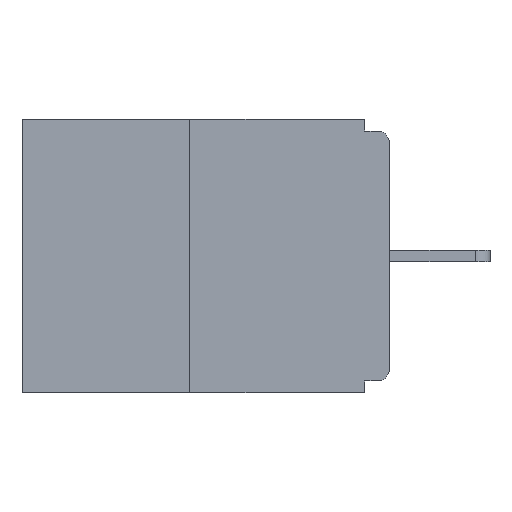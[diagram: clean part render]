
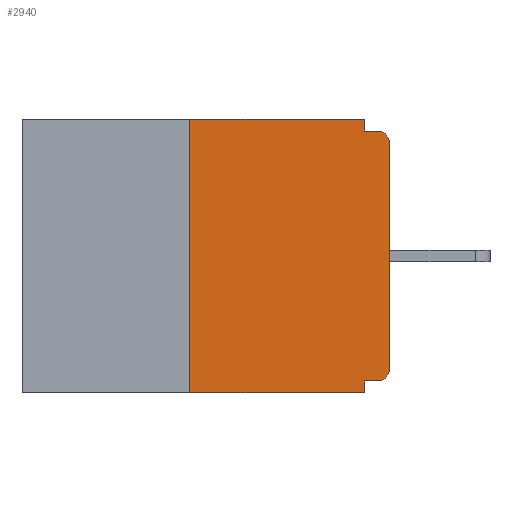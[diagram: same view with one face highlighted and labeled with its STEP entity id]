
A CAD part, left-side view. The second image highlights one B-rep face of the part: STEP entity #2940.
In plain terms, the highlighted planar face has unit normal (-1, 0, 0).
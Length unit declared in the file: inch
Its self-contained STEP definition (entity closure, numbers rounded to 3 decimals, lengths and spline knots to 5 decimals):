
#177 = FACE_OUTER_BOUND ( 'NONE', #659, .T. ) ;
#199 = CARTESIAN_POINT ( 'NONE',  ( 0., 0.015, -0.328 ) ) ;
#419 = CARTESIAN_POINT ( 'NONE',  ( 0., 0.031, 0. ) ) ;
#659 = EDGE_LOOP ( 'NONE', ( #4234, #4294, #4307, #4399, #4528, #4641, #4643, #4675, #4744, #4788 ) ) ;
#660 = VECTOR ( 'NONE', #5358, 39.37008 ) ;
#672 = VECTOR ( 'NONE', #8830, 39.37008 ) ;
#677 = LINE ( 'NONE', #7534, #672 ) ;
#694 = LINE ( 'NONE', #4751, #660 ) ;
#746 = VECTOR ( 'NONE', #3418, 39.37008 ) ;
#864 = LINE ( 'NONE', #7514, #746 ) ;
#878 = VECTOR ( 'NONE', #9875, 39.37008 ) ;
#987 = AXIS2_PLACEMENT_3D ( 'NONE', #4759, #5664, #1078 ) ;
#1072 = LINE ( 'NONE', #3291, #878 ) ;
#1078 = DIRECTION ( 'NONE',  ( 0., 0., -1. ) ) ;
#1327 = PLANE ( 'NONE',  #10338 ) ;
#1788 = VERTEX_POINT ( 'NONE', #419 ) ;
#1870 = EDGE_CURVE ( 'NONE', #2166, #1788, #6035, .T. ) ;
#2054 = EDGE_CURVE ( 'NONE', #8204, #8087, #4799, .T. ) ;
#2150 = EDGE_CURVE ( 'NONE', #7893, #8150, #4353, .T. ) ;
#2166 = VERTEX_POINT ( 'NONE', #4465 ) ;
#2228 = EDGE_CURVE ( 'NONE', #7756, #8025, #4148, .T. ) ;
#2294 = EDGE_CURVE ( 'NONE', #7893, #8204, #3614, .T. ) ;
#2298 = CARTESIAN_POINT ( 'NONE',  ( 0., 0., -0.328 ) ) ;
#2368 = EDGE_CURVE ( 'NONE', #8087, #8025, #3404, .T. ) ;
#2396 = DIRECTION ( 'NONE',  ( 0., -1., 0. ) ) ;
#2397 = CARTESIAN_POINT ( 'NONE',  ( 0., 0.46, 0. ) ) ;
#2735 = CARTESIAN_POINT ( 'NONE',  ( 0., 0.031, -0.015 ) ) ;
#2753 = EDGE_CURVE ( 'NONE', #7722, #2166, #1072, .T. ) ;
#2779 = EDGE_CURVE ( 'NONE', #7722, #3634, #864, .T. ) ;
#2795 = EDGE_CURVE ( 'NONE', #8150, #3634, #677, .T. ) ;
#2811 = EDGE_CURVE ( 'NONE', #1788, #7756, #694, .T. ) ;
#2940 = ADVANCED_FACE ( 'NONE', ( #177 ), #1327, .F. ) ;
#3130 = CARTESIAN_POINT ( 'NONE',  ( 0., 0.25, -0.343 ) ) ;
#3291 = CARTESIAN_POINT ( 'NONE',  ( 0., 0.25, 0. ) ) ;
#3404 = CIRCLE ( 'NONE', #987, 0.015 ) ;
#3418 = DIRECTION ( 'NONE',  ( 0., -1., 0. ) ) ;
#3599 = DIRECTION ( 'NONE',  ( 0., 1., 0. ) ) ;
#3601 = CARTESIAN_POINT ( 'NONE',  ( 0., 0., -0.313 ) ) ;
#3614 = CIRCLE ( 'NONE', #9066, 0.015 ) ;
#3634 = VERTEX_POINT ( 'NONE', #5076 ) ;
#3985 = VECTOR ( 'NONE', #5439, 39.37008 ) ;
#4148 = LINE ( 'NONE', #5165, #3985 ) ;
#4234 = ORIENTED_EDGE ( 'NONE', *, *, #1870, .F. ) ;
#4284 = VECTOR ( 'NONE', #3599, 39.37008 ) ;
#4294 = ORIENTED_EDGE ( 'NONE', *, *, #2753, .F. ) ;
#4307 = ORIENTED_EDGE ( 'NONE', *, *, #2779, .T. ) ;
#4353 = LINE ( 'NONE', #2298, #4284 ) ;
#4399 = ORIENTED_EDGE ( 'NONE', *, *, #2795, .F. ) ;
#4465 = CARTESIAN_POINT ( 'NONE',  ( 0., 0.25, 0. ) ) ;
#4528 = ORIENTED_EDGE ( 'NONE', *, *, #2150, .F. ) ;
#4636 = DIRECTION ( 'NONE',  ( 1., 0., 0. ) ) ;
#4641 = ORIENTED_EDGE ( 'NONE', *, *, #2294, .T. ) ;
#4643 = ORIENTED_EDGE ( 'NONE', *, *, #2054, .T. ) ;
#4675 = ORIENTED_EDGE ( 'NONE', *, *, #2368, .T. ) ;
#4744 = ORIENTED_EDGE ( 'NONE', *, *, #2228, .F. ) ;
#4751 = CARTESIAN_POINT ( 'NONE',  ( 0., 0.031, 0. ) ) ;
#4759 = CARTESIAN_POINT ( 'NONE',  ( 0., 0.015, -0.03 ) ) ;
#4788 = ORIENTED_EDGE ( 'NONE', *, *, #2811, .F. ) ;
#4799 = LINE ( 'NONE', #7427, #5336 ) ;
#5076 = CARTESIAN_POINT ( 'NONE',  ( 0., 0.031, -0.343 ) ) ;
#5165 = CARTESIAN_POINT ( 'NONE',  ( 0., 0., -0.015 ) ) ;
#5200 = CARTESIAN_POINT ( 'NONE',  ( 0., 0., -0.03 ) ) ;
#5336 = VECTOR ( 'NONE', #6385, 39.37008 ) ;
#5358 = DIRECTION ( 'NONE',  ( 0., 0., -1. ) ) ;
#5439 = DIRECTION ( 'NONE',  ( 0., -1., 0. ) ) ;
#5664 = DIRECTION ( 'NONE',  ( -1., 0., 0. ) ) ;
#6035 = LINE ( 'NONE', #2397, #6055 ) ;
#6055 = VECTOR ( 'NONE', #2396, 39.37008 ) ;
#6385 = DIRECTION ( 'NONE',  ( 0., 0., 1. ) ) ;
#6772 = DIRECTION ( 'NONE',  ( 0., 0., -1. ) ) ;
#7427 = CARTESIAN_POINT ( 'NONE',  ( 0., 0., 0. ) ) ;
#7514 = CARTESIAN_POINT ( 'NONE',  ( 0., 0.46, -0.343 ) ) ;
#7534 = CARTESIAN_POINT ( 'NONE',  ( 0., 0.031, -0.343 ) ) ;
#7722 = VERTEX_POINT ( 'NONE', #3130 ) ;
#7756 = VERTEX_POINT ( 'NONE', #2735 ) ;
#7888 = DIRECTION ( 'NONE',  ( 0., 0., -1. ) ) ;
#7893 = VERTEX_POINT ( 'NONE', #199 ) ;
#8025 = VERTEX_POINT ( 'NONE', #8805 ) ;
#8087 = VERTEX_POINT ( 'NONE', #5200 ) ;
#8150 = VERTEX_POINT ( 'NONE', #8358 ) ;
#8204 = VERTEX_POINT ( 'NONE', #3601 ) ;
#8358 = CARTESIAN_POINT ( 'NONE',  ( 0., 0.031, -0.328 ) ) ;
#8456 = DIRECTION ( 'NONE',  ( -1., 0., 0. ) ) ;
#8512 = CARTESIAN_POINT ( 'NONE',  ( 0., 0.015, -0.313 ) ) ;
#8805 = CARTESIAN_POINT ( 'NONE',  ( 0., 0.015, -0.015 ) ) ;
#8830 = DIRECTION ( 'NONE',  ( 0., 0., -1. ) ) ;
#9066 = AXIS2_PLACEMENT_3D ( 'NONE', #8512, #8456, #7888 ) ;
#9472 = CARTESIAN_POINT ( 'NONE',  ( 0., 0.46, 0. ) ) ;
#9875 = DIRECTION ( 'NONE',  ( 0., 0., 1. ) ) ;
#10338 = AXIS2_PLACEMENT_3D ( 'NONE', #9472, #4636, #6772 ) ;
